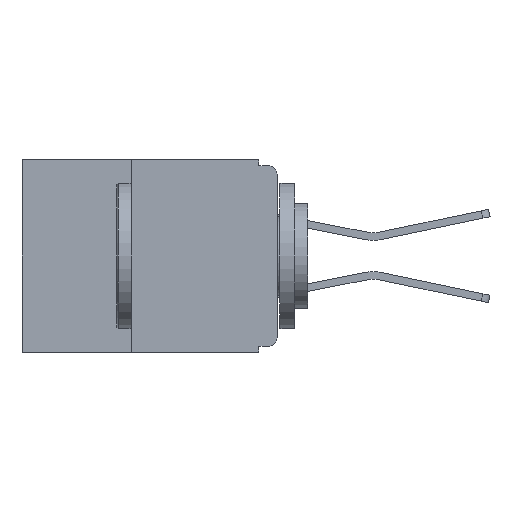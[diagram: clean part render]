
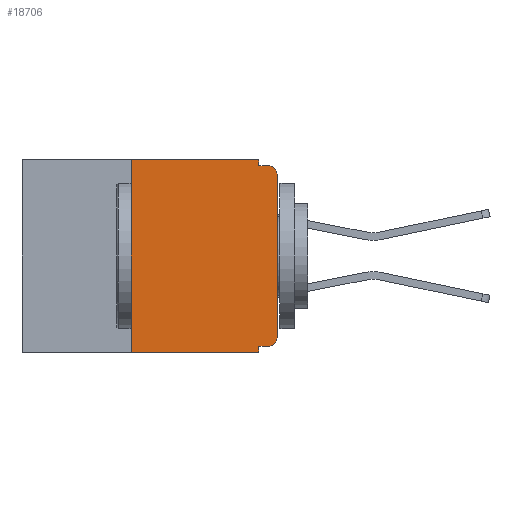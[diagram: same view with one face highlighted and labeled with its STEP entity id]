
A CAD part, left-side view. The second image highlights one B-rep face of the part: STEP entity #18706.
In plain terms, the highlighted planar face has unit normal (-1, 0, 0).
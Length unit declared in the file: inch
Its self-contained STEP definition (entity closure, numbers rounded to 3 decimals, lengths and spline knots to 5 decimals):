
#436 = FACE_OUTER_BOUND ( 'NONE', #14813, .T. ) ;
#696 = ORIENTED_EDGE ( 'NONE', *, *, #25832, .F. ) ;
#1365 = ORIENTED_EDGE ( 'NONE', *, *, #24416, .T. ) ;
#1599 = EDGE_CURVE ( 'NONE', #18166, #28140, #22690, .T. ) ;
#2430 = DIRECTION ( 'NONE',  ( 0., 1., 0. ) ) ;
#3073 = CARTESIAN_POINT ( 'NONE',  ( 0., 0.031, 0. ) ) ;
#3874 = LINE ( 'NONE', #20245, #26428 ) ;
#3992 = VERTEX_POINT ( 'NONE', #27500 ) ;
#4595 = CARTESIAN_POINT ( 'NONE',  ( 0., 0.437, 0. ) ) ;
#4928 = VERTEX_POINT ( 'NONE', #13450 ) ;
#5548 = CARTESIAN_POINT ( 'NONE',  ( 0., 0.25, -0.33 ) ) ;
#5889 = VERTEX_POINT ( 'NONE', #11953 ) ;
#6097 = LINE ( 'NONE', #19489, #22869 ) ;
#6334 = DIRECTION ( 'NONE',  ( 0., 0., 1. ) ) ;
#6350 = ORIENTED_EDGE ( 'NONE', *, *, #21552, .F. ) ;
#6913 = EDGE_CURVE ( 'NONE', #5889, #4928, #18429, .T. ) ;
#7180 = DIRECTION ( 'NONE',  ( -1., 0., 0. ) ) ;
#7184 = DIRECTION ( 'NONE',  ( 0., 0., -1. ) ) ;
#7509 = LINE ( 'NONE', #10072, #13340 ) ;
#7544 = DIRECTION ( 'NONE',  ( 0., 0., -1. ) ) ;
#7589 = ORIENTED_EDGE ( 'NONE', *, *, #17944, .T. ) ;
#8263 = LINE ( 'NONE', #12488, #24985 ) ;
#9155 = ORIENTED_EDGE ( 'NONE', *, *, #27229, .F. ) ;
#9629 = LINE ( 'NONE', #25010, #20628 ) ;
#9735 = ORIENTED_EDGE ( 'NONE', *, *, #10536, .F. ) ;
#10072 = CARTESIAN_POINT ( 'NONE',  ( 0., 0., 0. ) ) ;
#10513 = PLANE ( 'NONE',  #20525 ) ;
#10536 = EDGE_CURVE ( 'NONE', #3992, #22436, #8263, .T. ) ;
#10779 = ORIENTED_EDGE ( 'NONE', *, *, #6913, .F. ) ;
#11060 = VECTOR ( 'NONE', #2430, 39.37008 ) ;
#11443 = AXIS2_PLACEMENT_3D ( 'NONE', #20330, #7180, #22483 ) ;
#11838 = VECTOR ( 'NONE', #17812, 39.37008 ) ;
#11953 = CARTESIAN_POINT ( 'NONE',  ( 0., 0.25, 0. ) ) ;
#12488 = CARTESIAN_POINT ( 'NONE',  ( 0., 0., -0.01 ) ) ;
#12715 = DIRECTION ( 'NONE',  ( 1., 0., 0. ) ) ;
#13026 = CARTESIAN_POINT ( 'NONE',  ( 0., 0.015, -0.32 ) ) ;
#13130 = DIRECTION ( 'NONE',  ( -1., 0., 0. ) ) ;
#13247 = CARTESIAN_POINT ( 'NONE',  ( 0., 0., -0.32 ) ) ;
#13340 = VECTOR ( 'NONE', #25322, 39.37008 ) ;
#13450 = CARTESIAN_POINT ( 'NONE',  ( 0., 0.031, 0. ) ) ;
#14615 = CIRCLE ( 'NONE', #17125, 0.015 ) ;
#14698 = VERTEX_POINT ( 'NONE', #27098 ) ;
#14742 = DIRECTION ( 'NONE',  ( 0., -1., 0. ) ) ;
#14813 = EDGE_LOOP ( 'NONE', ( #7589, #26983, #9735, #9155, #10779, #696, #1365, #6350, #14850, #16396 ) ) ;
#14850 = ORIENTED_EDGE ( 'NONE', *, *, #1599, .F. ) ;
#16332 = DIRECTION ( 'NONE',  ( 0., -1., 0. ) ) ;
#16396 = ORIENTED_EDGE ( 'NONE', *, *, #21385, .T. ) ;
#17073 = LINE ( 'NONE', #3073, #22152 ) ;
#17125 = AXIS2_PLACEMENT_3D ( 'NONE', #26139, #13130, #28233 ) ;
#17812 = DIRECTION ( 'NONE',  ( 0., -1., 0. ) ) ;
#17944 = EDGE_CURVE ( 'NONE', #27439, #14698, #7509, .T. ) ;
#18166 = VERTEX_POINT ( 'NONE', #13026 ) ;
#18429 = LINE ( 'NONE', #4595, #11838 ) ;
#18706 = ADVANCED_FACE ( 'NONE', ( #436 ), #10513, .F. ) ;
#19489 = CARTESIAN_POINT ( 'NONE',  ( 0., 0.25, -0.33 ) ) ;
#20245 = CARTESIAN_POINT ( 'NONE',  ( 0., 0.031, -0.33 ) ) ;
#20330 = CARTESIAN_POINT ( 'NONE',  ( 0., 0.015, -0.025 ) ) ;
#20525 = AXIS2_PLACEMENT_3D ( 'NONE', #21452, #12715, #27834 ) ;
#20627 = VERTEX_POINT ( 'NONE', #27730 ) ;
#20628 = VECTOR ( 'NONE', #16332, 39.37008 ) ;
#21385 = EDGE_CURVE ( 'NONE', #18166, #27439, #14615, .T. ) ;
#21442 = CARTESIAN_POINT ( 'NONE',  ( 0., 0., -0.305 ) ) ;
#21452 = CARTESIAN_POINT ( 'NONE',  ( 0., 0.437, 0. ) ) ;
#21552 = EDGE_CURVE ( 'NONE', #28140, #20627, #3874, .T. ) ;
#22152 = VECTOR ( 'NONE', #7544, 39.37008 ) ;
#22436 = VERTEX_POINT ( 'NONE', #27625 ) ;
#22483 = DIRECTION ( 'NONE',  ( 0., 0., -1. ) ) ;
#22690 = LINE ( 'NONE', #13247, #11060 ) ;
#22869 = VECTOR ( 'NONE', #6334, 39.37008 ) ;
#22954 = VERTEX_POINT ( 'NONE', #5548 ) ;
#23820 = CARTESIAN_POINT ( 'NONE',  ( 0., 0.031, -0.32 ) ) ;
#24245 = EDGE_CURVE ( 'NONE', #14698, #22436, #24269, .T. ) ;
#24269 = CIRCLE ( 'NONE', #11443, 0.015 ) ;
#24416 = EDGE_CURVE ( 'NONE', #22954, #20627, #9629, .T. ) ;
#24985 = VECTOR ( 'NONE', #14742, 39.37008 ) ;
#25010 = CARTESIAN_POINT ( 'NONE',  ( 0., 0.437, -0.33 ) ) ;
#25322 = DIRECTION ( 'NONE',  ( 0., 0., 1. ) ) ;
#25832 = EDGE_CURVE ( 'NONE', #22954, #5889, #6097, .T. ) ;
#26139 = CARTESIAN_POINT ( 'NONE',  ( 0., 0.015, -0.305 ) ) ;
#26428 = VECTOR ( 'NONE', #7184, 39.37008 ) ;
#26983 = ORIENTED_EDGE ( 'NONE', *, *, #24245, .T. ) ;
#27098 = CARTESIAN_POINT ( 'NONE',  ( 0., 0., -0.025 ) ) ;
#27229 = EDGE_CURVE ( 'NONE', #4928, #3992, #17073, .T. ) ;
#27439 = VERTEX_POINT ( 'NONE', #21442 ) ;
#27500 = CARTESIAN_POINT ( 'NONE',  ( 0., 0.031, -0.01 ) ) ;
#27625 = CARTESIAN_POINT ( 'NONE',  ( 0., 0.015, -0.01 ) ) ;
#27730 = CARTESIAN_POINT ( 'NONE',  ( 0., 0.031, -0.33 ) ) ;
#27834 = DIRECTION ( 'NONE',  ( 0., 0., -1. ) ) ;
#28140 = VERTEX_POINT ( 'NONE', #23820 ) ;
#28233 = DIRECTION ( 'NONE',  ( 0., 0., -1. ) ) ;
